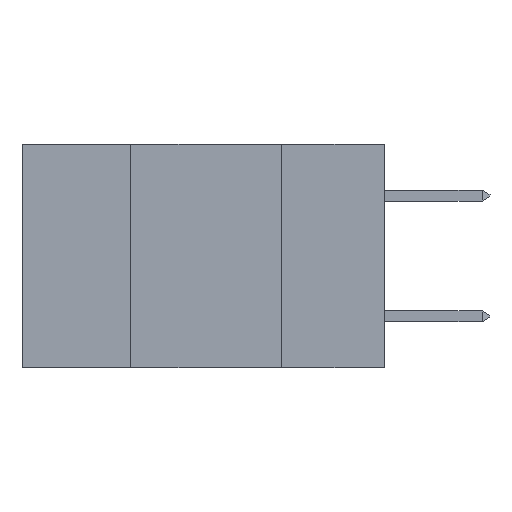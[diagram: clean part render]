
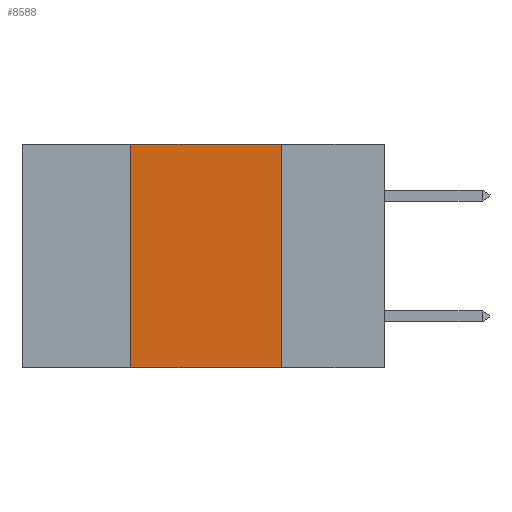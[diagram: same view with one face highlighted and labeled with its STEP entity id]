
A CAD part, left-side view. The second image highlights one B-rep face of the part: STEP entity #8588.
In plain terms, the highlighted planar face has unit normal (-1, 0, 0).
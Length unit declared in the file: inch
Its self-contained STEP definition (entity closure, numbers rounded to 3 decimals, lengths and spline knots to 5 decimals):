
#313 = DIRECTION ( 'NONE',  ( 0., 0., -1. ) ) ;
#556 = DIRECTION ( 'NONE',  ( 0., 0., 1. ) ) ;
#1046 = VECTOR ( 'NONE', #556, 39.37008 ) ;
#2067 = CARTESIAN_POINT ( 'NONE',  ( 0., 0.6, 0. ) ) ;
#2262 = EDGE_CURVE ( 'NONE', #3461, #5890, #8722, .T. ) ;
#3086 = DIRECTION ( 'NONE',  ( 0., 0., -1. ) ) ;
#3442 = LINE ( 'NONE', #11359, #8451 ) ;
#3461 = VERTEX_POINT ( 'NONE', #5002 ) ;
#3527 = CARTESIAN_POINT ( 'NONE',  ( 0., 0.42, 0. ) ) ;
#3827 = LINE ( 'NONE', #5882, #8541 ) ;
#4198 = VERTEX_POINT ( 'NONE', #7321 ) ;
#4551 = EDGE_CURVE ( 'NONE', #4198, #11945, #11674, .T. ) ;
#4951 = PLANE ( 'NONE',  #11908 ) ;
#5002 = CARTESIAN_POINT ( 'NONE',  ( 0., 0.42, -0.37 ) ) ;
#5795 = VECTOR ( 'NONE', #313, 39.37008 ) ;
#5882 = CARTESIAN_POINT ( 'NONE',  ( 0., 0.6, -0.37 ) ) ;
#5890 = VERTEX_POINT ( 'NONE', #3527 ) ;
#6015 = FACE_OUTER_BOUND ( 'NONE', #10745, .T. ) ;
#6862 = ORIENTED_EDGE ( 'NONE', *, *, #11587, .F. ) ;
#6866 = DIRECTION ( 'NONE',  ( 0., -1., 0. ) ) ;
#7321 = CARTESIAN_POINT ( 'NONE',  ( 0., 0.17, 0. ) ) ;
#7658 = DIRECTION ( 'NONE',  ( 0., -1., 0. ) ) ;
#8451 = VECTOR ( 'NONE', #7658, 39.37008 ) ;
#8541 = VECTOR ( 'NONE', #6866, 39.37008 ) ;
#8560 = EDGE_CURVE ( 'NONE', #3461, #11945, #3827, .T. ) ;
#8588 = ADVANCED_FACE ( 'NONE', ( #6015 ), #4951, .F. ) ;
#8722 = LINE ( 'NONE', #12003, #1046 ) ;
#8748 = DIRECTION ( 'NONE',  ( 1., 0., 0. ) ) ;
#9486 = ORIENTED_EDGE ( 'NONE', *, *, #2262, .F. ) ;
#10745 = EDGE_LOOP ( 'NONE', ( #12225, #6862, #9486, #10888 ) ) ;
#10851 = CARTESIAN_POINT ( 'NONE',  ( 0., 0.17, -0.37 ) ) ;
#10888 = ORIENTED_EDGE ( 'NONE', *, *, #8560, .T. ) ;
#11359 = CARTESIAN_POINT ( 'NONE',  ( 0., 0.6, 0. ) ) ;
#11587 = EDGE_CURVE ( 'NONE', #5890, #4198, #3442, .T. ) ;
#11674 = LINE ( 'NONE', #12414, #5795 ) ;
#11908 = AXIS2_PLACEMENT_3D ( 'NONE', #2067, #8748, #3086 ) ;
#11945 = VERTEX_POINT ( 'NONE', #10851 ) ;
#12003 = CARTESIAN_POINT ( 'NONE',  ( 0., 0.42, 0. ) ) ;
#12225 = ORIENTED_EDGE ( 'NONE', *, *, #4551, .F. ) ;
#12414 = CARTESIAN_POINT ( 'NONE',  ( 0., 0.17, 0. ) ) ;
